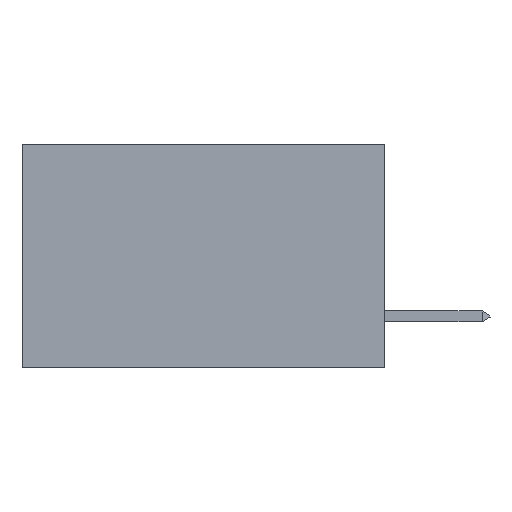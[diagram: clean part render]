
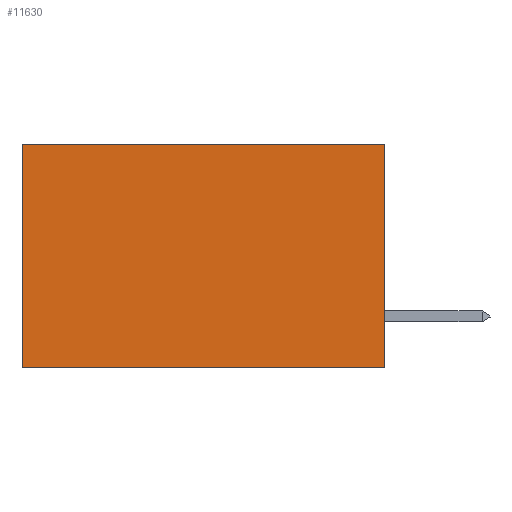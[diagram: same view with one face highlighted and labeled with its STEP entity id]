
A CAD part, left-side view. The second image highlights one B-rep face of the part: STEP entity #11630.
In plain terms, the highlighted planar face has unit normal (-1, 0, 0).
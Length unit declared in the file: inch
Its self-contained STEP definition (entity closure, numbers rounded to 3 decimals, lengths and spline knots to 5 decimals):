
#405 = DIRECTION ( 'NONE',  ( 1., 0., 0. ) ) ;
#1708 = EDGE_LOOP ( 'NONE', ( #20274, #12101, #3257, #5698 ) ) ;
#2117 = FACE_OUTER_BOUND ( 'NONE', #1708, .T. ) ;
#2150 = EDGE_CURVE ( 'NONE', #10427, #4550, #17222, .T. ) ;
#3257 = ORIENTED_EDGE ( 'NONE', *, *, #2150, .F. ) ;
#3985 = CARTESIAN_POINT ( 'NONE',  ( 0.2875, 0., -0.37 ) ) ;
#4277 = VERTEX_POINT ( 'NONE', #16740 ) ;
#4550 = VERTEX_POINT ( 'NONE', #5612 ) ;
#4770 = LINE ( 'NONE', #6199, #13164 ) ;
#5612 = CARTESIAN_POINT ( 'NONE',  ( 0.2875, 0., -0.37 ) ) ;
#5662 = DIRECTION ( 'NONE',  ( 0., 1., 0. ) ) ;
#5698 = ORIENTED_EDGE ( 'NONE', *, *, #20687, .T. ) ;
#5705 = VERTEX_POINT ( 'NONE', #18823 ) ;
#5712 = AXIS2_PLACEMENT_3D ( 'NONE', #17082, #405, #12238 ) ;
#6199 = CARTESIAN_POINT ( 'NONE',  ( 0.2875, 0., 0. ) ) ;
#7662 = EDGE_CURVE ( 'NONE', #4277, #5705, #12573, .T. ) ;
#7900 = DIRECTION ( 'NONE',  ( 0., 1., 0. ) ) ;
#10427 = VERTEX_POINT ( 'NONE', #16589 ) ;
#11630 = ADVANCED_FACE ( 'NONE', ( #2117 ), #18708, .F. ) ;
#12051 = VECTOR ( 'NONE', #17484, 39.37008 ) ;
#12101 = ORIENTED_EDGE ( 'NONE', *, *, #14490, .F. ) ;
#12113 = VECTOR ( 'NONE', #5662, 39.37008 ) ;
#12238 = DIRECTION ( 'NONE',  ( 0., 0., -1. ) ) ;
#12573 = LINE ( 'NONE', #19113, #12051 ) ;
#12879 = VECTOR ( 'NONE', #16323, 39.37008 ) ;
#13164 = VECTOR ( 'NONE', #7900, 39.37008 ) ;
#14490 = EDGE_CURVE ( 'NONE', #4550, #5705, #16435, .T. ) ;
#14764 = CARTESIAN_POINT ( 'NONE',  ( 0.2875, 0., 0. ) ) ;
#16323 = DIRECTION ( 'NONE',  ( 0., 0., -1. ) ) ;
#16435 = LINE ( 'NONE', #3985, #12113 ) ;
#16589 = CARTESIAN_POINT ( 'NONE',  ( 0.2875, 0., 0. ) ) ;
#16740 = CARTESIAN_POINT ( 'NONE',  ( 0.2875, 0.6, 0. ) ) ;
#17082 = CARTESIAN_POINT ( 'NONE',  ( 0.2875, 0., 0. ) ) ;
#17222 = LINE ( 'NONE', #14764, #12879 ) ;
#17484 = DIRECTION ( 'NONE',  ( 0., 0., -1. ) ) ;
#18708 = PLANE ( 'NONE',  #5712 ) ;
#18823 = CARTESIAN_POINT ( 'NONE',  ( 0.2875, 0.6, -0.37 ) ) ;
#19113 = CARTESIAN_POINT ( 'NONE',  ( 0.2875, 0.6, 0. ) ) ;
#20274 = ORIENTED_EDGE ( 'NONE', *, *, #7662, .T. ) ;
#20687 = EDGE_CURVE ( 'NONE', #10427, #4277, #4770, .T. ) ;
